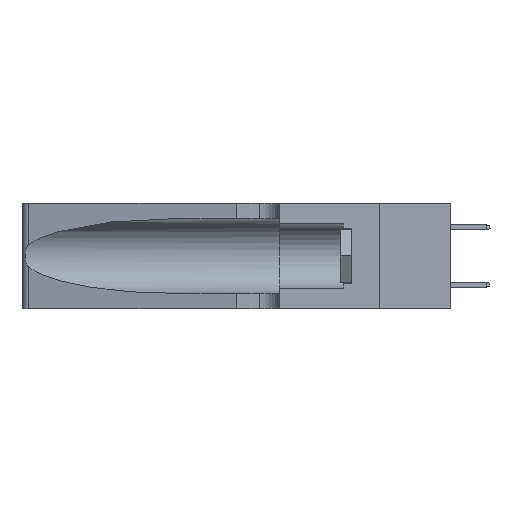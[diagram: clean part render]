
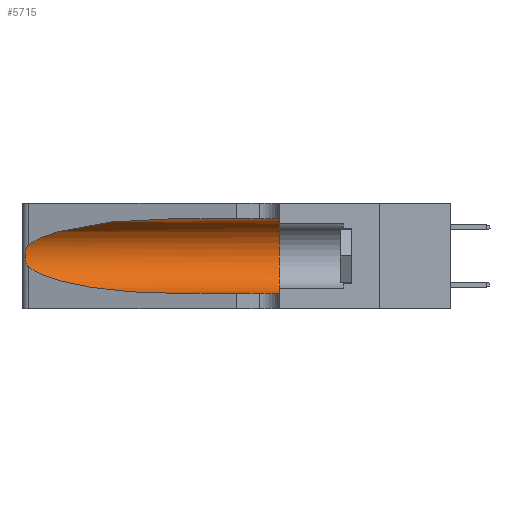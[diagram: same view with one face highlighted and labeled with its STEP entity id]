
A CAD part, left-side view. The second image highlights one B-rep face of the part: STEP entity #5715.
In plain terms, the highlighted cylindrical face has radius 3.308 mm (diameter 6.617 mm), a partial arc.
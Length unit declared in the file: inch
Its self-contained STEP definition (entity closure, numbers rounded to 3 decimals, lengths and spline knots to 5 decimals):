
#313 = CARTESIAN_POINT ( 'NONE',  ( 0.1305, 0.72297, 0.05475 ) ) ;
#344 = EDGE_CURVE ( 'NONE', #11365, #17921, #10707, .T. ) ;
#676 = CARTESIAN_POINT ( 'NONE',  ( 0.25487, 1.22718, 0.22369 ) ) ;
#782 = CARTESIAN_POINT ( 'NONE',  ( 0.25555, 1.22993, 0.14849 ) ) ;
#1548 = CARTESIAN_POINT ( 'NONE',  ( 0.1305, 1.61858, 0.31525 ) ) ;
#1606 = CARTESIAN_POINT ( 'NONE',  ( 0.1305, 1.61858, 0.05475 ) ) ;
#1607 = DIRECTION ( 'NONE',  ( 0., -1., 0. ) ) ;
#1800 = LINE ( 'NONE', #1606, #4335 ) ;
#1953 = DIRECTION ( 'NONE',  ( 0., 0., 1. ) ) ;
#2224 = CARTESIAN_POINT ( 'NONE',  ( 0.25487, 1.22718, 0.14631 ) ) ;
#2251 = CARTESIAN_POINT ( 'NONE',  ( 0.1305, 0.35, 0.31525 ) ) ;
#2418 = CARTESIAN_POINT ( 'NONE',  ( 0.26018, 1.23835, 0.19895 ) ) ;
#3392 = DIRECTION ( 'NONE',  ( 0., 1., 0. ) ) ;
#3420 = CARTESIAN_POINT ( 'NONE',  ( 0.25487, 1.22718, 0.14631 ) ) ;
#3443 = VERTEX_POINT ( 'NONE', #313 ) ;
#4056 = CARTESIAN_POINT ( 'NONE',  ( 0.25856, 1.23593, 0.16098 ) ) ;
#4124 = CARTESIAN_POINT ( 'NONE',  ( 0.25487, 1.22718, 0.14631 ) ) ;
#4335 = VECTOR ( 'NONE', #9213, 39.37008 ) ;
#4687 = FACE_OUTER_BOUND ( 'NONE', #11063, .T. ) ;
#4837 = CARTESIAN_POINT ( 'NONE',  ( 0.1305, 0.35, 0.185 ) ) ;
#4913 = CARTESIAN_POINT ( 'NONE',  ( 0.18966, 0.96281, 0.31525 ) ) ;
#5045 = CARTESIAN_POINT ( 'NONE',  ( 0.1305, 0.35, 0.05475 ) ) ;
#5156 = B_SPLINE_CURVE_WITH_KNOTS ( 'NONE', 3,
 ( #15750, #8480, #13953, #17119, #18542, #2418, #12816, #14236, #11294, #4056, #14327, #12905, #782, #2224 ),
 .UNSPECIFIED., .F., .F.,
 ( 4, 2, 2, 2, 2, 2, 4 ),
 ( 0., 0.00027, 0.00053, 0.00107, 0.0016, 0.00187, 0.00214 ),
 .UNSPECIFIED. ) ;
#5715 = ADVANCED_FACE ( 'NONE', ( #4687 ), #14763, .F. ) ;
#5951 = CIRCLE ( 'NONE', #17597, 0.13025 ) ;
#6083 = EDGE_CURVE ( 'NONE', #15223, #13887, #5951, .T. ) ;
#6407 = CARTESIAN_POINT ( 'NONE',  ( 0.18966, 0.96281, 0.05475 ) ) ;
#7189 = ORIENTED_EDGE ( 'NONE', *, *, #10344, .T. ) ;
#7496 = AXIS2_PLACEMENT_3D ( 'NONE', #10474, #1607, #10572 ) ;
#7816 = CARTESIAN_POINT ( 'NONE',  ( 0.2373, 1.15595, 0.28018 ) ) ;
#7950 = CARTESIAN_POINT ( 'NONE',  ( 0.1305, 0.72297, 0.05475 ) ) ;
#8069 = CARTESIAN_POINT ( 'NONE',  ( 0.25487, 1.22718, 0.22369 ) ) ;
#8125 = EDGE_CURVE ( 'NONE', #11365, #15223, #17692, .T. ) ;
#8380 = CARTESIAN_POINT ( 'NONE',  ( 0.1305, 0.72297, 0.31525 ) ) ;
#8480 = CARTESIAN_POINT ( 'NONE',  ( 0.25555, 1.22994, 0.2215 ) ) ;
#8573 = ORIENTED_EDGE ( 'NONE', *, *, #16977, .T. ) ;
#8730 = ORIENTED_EDGE ( 'NONE', *, *, #6083, .F. ) ;
#9213 = DIRECTION ( 'NONE',  ( 0., -1., 0. ) ) ;
#9385 = CARTESIAN_POINT ( 'NONE',  ( 0.2373, 1.15595, 0.08982 ) ) ;
#9724 = EDGE_CURVE ( 'NONE', #17921, #14474, #5156, .T. ) ;
#10344 = EDGE_CURVE ( 'NONE', #3443, #13887, #1800, .T. ) ;
#10356 = ORIENTED_EDGE ( 'NONE', *, *, #9724, .T. ) ;
#10474 = CARTESIAN_POINT ( 'NONE',  ( 0.1305, 1.61858, 0.185 ) ) ;
#10572 = DIRECTION ( 'NONE',  ( 0., 0., -1. ) ) ;
#10707 =( BOUNDED_CURVE ( )  B_SPLINE_CURVE ( 3, ( #16816, #4913, #7816, #676 ),
 .UNSPECIFIED., .F., .T. ) 
 B_SPLINE_CURVE_WITH_KNOTS ( ( 4, 4 ),
 ( 1.5708, 2.84003 ),
 .UNSPECIFIED. ) 
 CURVE ( )  GEOMETRIC_REPRESENTATION_ITEM ( )  RATIONAL_B_SPLINE_CURVE ( ( 1., 0.87, 0.87, 1. ) ) 
 REPRESENTATION_ITEM ( '' )  );
#11063 = EDGE_LOOP ( 'NONE', ( #15053, #10356, #8573, #7189, #8730, #15824 ) ) ;
#11294 = CARTESIAN_POINT ( 'NONE',  ( 0.26017, 1.23833, 0.17102 ) ) ;
#11365 = VERTEX_POINT ( 'NONE', #8380 ) ;
#11945 =( BOUNDED_CURVE ( )  B_SPLINE_CURVE ( 3, ( #3420, #9385, #6407, #7950 ),
 .UNSPECIFIED., .F., .T. ) 
 B_SPLINE_CURVE_WITH_KNOTS ( ( 4, 4 ),
 ( 3.44316, 4.71239 ),
 .UNSPECIFIED. ) 
 CURVE ( )  GEOMETRIC_REPRESENTATION_ITEM ( )  RATIONAL_B_SPLINE_CURVE ( ( 1., 0.87, 0.87, 1. ) ) 
 REPRESENTATION_ITEM ( '' )  );
#12816 = CARTESIAN_POINT ( 'NONE',  ( 0.26075, 1.23896, 0.19203 ) ) ;
#12896 = VECTOR ( 'NONE', #16256, 39.37008 ) ;
#12905 = CARTESIAN_POINT ( 'NONE',  ( 0.25639, 1.23186, 0.15144 ) ) ;
#13887 = VERTEX_POINT ( 'NONE', #5045 ) ;
#13953 = CARTESIAN_POINT ( 'NONE',  ( 0.25639, 1.23184, 0.21858 ) ) ;
#14236 = CARTESIAN_POINT ( 'NONE',  ( 0.26075, 1.23896, 0.178 ) ) ;
#14327 = CARTESIAN_POINT ( 'NONE',  ( 0.25789, 1.23486, 0.15765 ) ) ;
#14474 = VERTEX_POINT ( 'NONE', #4124 ) ;
#14763 = CYLINDRICAL_SURFACE ( 'NONE', #7496, 0.13025 ) ;
#15053 = ORIENTED_EDGE ( 'NONE', *, *, #344, .T. ) ;
#15223 = VERTEX_POINT ( 'NONE', #2251 ) ;
#15750 = CARTESIAN_POINT ( 'NONE',  ( 0.25487, 1.22718, 0.22369 ) ) ;
#15824 = ORIENTED_EDGE ( 'NONE', *, *, #8125, .F. ) ;
#16256 = DIRECTION ( 'NONE',  ( 0., -1., 0. ) ) ;
#16816 = CARTESIAN_POINT ( 'NONE',  ( 0.1305, 0.72297, 0.31525 ) ) ;
#16977 = EDGE_CURVE ( 'NONE', #14474, #3443, #11945, .T. ) ;
#17119 = CARTESIAN_POINT ( 'NONE',  ( 0.25787, 1.23484, 0.2124 ) ) ;
#17597 = AXIS2_PLACEMENT_3D ( 'NONE', #4837, #3392, #1953 ) ;
#17692 = LINE ( 'NONE', #1548, #12896 ) ;
#17921 = VERTEX_POINT ( 'NONE', #8069 ) ;
#18542 = CARTESIAN_POINT ( 'NONE',  ( 0.25854, 1.2359, 0.20912 ) ) ;
